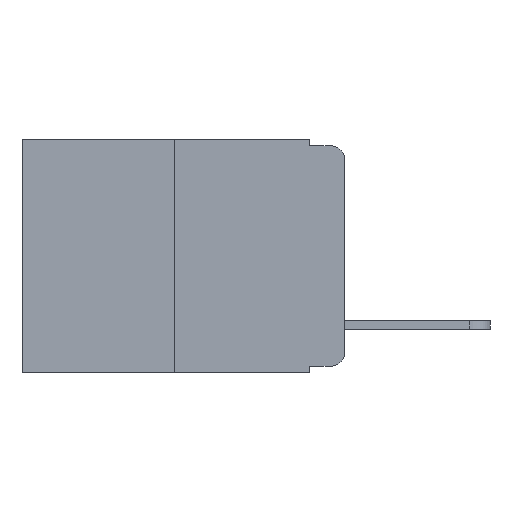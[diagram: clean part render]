
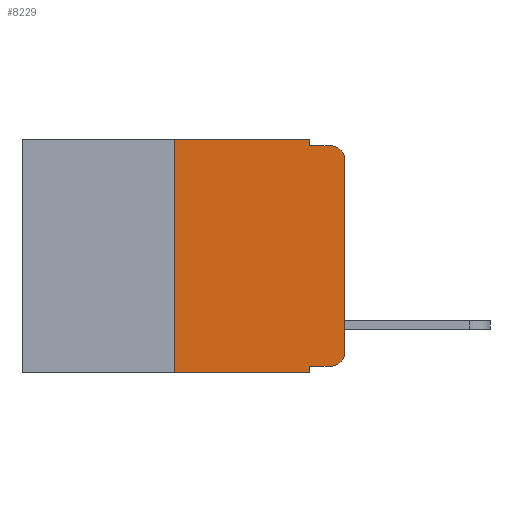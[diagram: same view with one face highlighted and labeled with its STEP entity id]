
A CAD part, left-side view. The second image highlights one B-rep face of the part: STEP entity #8229.
In plain terms, the highlighted planar face has unit normal (-1, 0, 0).
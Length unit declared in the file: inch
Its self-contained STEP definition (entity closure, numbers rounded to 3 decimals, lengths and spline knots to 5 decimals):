
#156 = EDGE_CURVE ( 'NONE', #7094, #14246, #8089, .T. ) ;
#465 = AXIS2_PLACEMENT_3D ( 'NONE', #5939, #7068, #10339 ) ;
#545 = VERTEX_POINT ( 'NONE', #8440 ) ;
#773 = CARTESIAN_POINT ( 'NONE',  ( 0., 0., -0.313 ) ) ;
#799 = VECTOR ( 'NONE', #7182, 39.37008 ) ;
#1074 = ORIENTED_EDGE ( 'NONE', *, *, #1769, .T. ) ;
#1079 = CARTESIAN_POINT ( 'NONE',  ( 0., 0.25, -0.343 ) ) ;
#1529 = EDGE_CURVE ( 'NONE', #7950, #545, #6477, .T. ) ;
#1769 = EDGE_CURVE ( 'NONE', #13994, #12586, #9266, .T. ) ;
#2109 = CARTESIAN_POINT ( 'NONE',  ( 0., 0.473, 0. ) ) ;
#2156 = DIRECTION ( 'NONE',  ( 0., -1., 0. ) ) ;
#2296 = LINE ( 'NONE', #3950, #11713 ) ;
#2600 = DIRECTION ( 'NONE',  ( 0., -1., 0. ) ) ;
#2976 = LINE ( 'NONE', #9887, #11186 ) ;
#3280 = DIRECTION ( 'NONE',  ( 0., 0., -1. ) ) ;
#3608 = DIRECTION ( 'NONE',  ( 0., 0., -1. ) ) ;
#3950 = CARTESIAN_POINT ( 'NONE',  ( 0., 0.25, 0. ) ) ;
#4275 = ORIENTED_EDGE ( 'NONE', *, *, #14229, .F. ) ;
#4282 = ORIENTED_EDGE ( 'NONE', *, *, #156, .F. ) ;
#4387 = CARTESIAN_POINT ( 'NONE',  ( 0., 0.051, 0. ) ) ;
#4635 = VERTEX_POINT ( 'NONE', #8736 ) ;
#4652 = EDGE_CURVE ( 'NONE', #545, #7094, #5763, .T. ) ;
#4872 = DIRECTION ( 'NONE',  ( 0., 0., 1. ) ) ;
#4906 = DIRECTION ( 'NONE',  ( 0., 0., 1. ) ) ;
#5021 = CARTESIAN_POINT ( 'NONE',  ( 0., 0.051, -0.333 ) ) ;
#5056 = EDGE_CURVE ( 'NONE', #12586, #4635, #2976, .T. ) ;
#5356 = PLANE ( 'NONE',  #9702 ) ;
#5615 = DIRECTION ( 'NONE',  ( 0., 0., -1. ) ) ;
#5763 = LINE ( 'NONE', #4387, #7341 ) ;
#5784 = CARTESIAN_POINT ( 'NONE',  ( 0., 0.02, -0.03 ) ) ;
#5939 = CARTESIAN_POINT ( 'NONE',  ( 0., 0.02, -0.313 ) ) ;
#6159 = ORIENTED_EDGE ( 'NONE', *, *, #5056, .T. ) ;
#6477 = LINE ( 'NONE', #2109, #11557 ) ;
#6562 = CARTESIAN_POINT ( 'NONE',  ( 0., 0.051, -0.343 ) ) ;
#6568 = ORIENTED_EDGE ( 'NONE', *, *, #7954, .T. ) ;
#6570 = EDGE_CURVE ( 'NONE', #4635, #14246, #12740, .T. ) ;
#7065 = VERTEX_POINT ( 'NONE', #6562 ) ;
#7068 = DIRECTION ( 'NONE',  ( -1., 0., 0. ) ) ;
#7094 = VERTEX_POINT ( 'NONE', #13340 ) ;
#7182 = DIRECTION ( 'NONE',  ( 0., -1., 0. ) ) ;
#7341 = VECTOR ( 'NONE', #11244, 39.37008 ) ;
#7663 = ORIENTED_EDGE ( 'NONE', *, *, #6570, .T. ) ;
#7739 = VECTOR ( 'NONE', #9499, 39.37008 ) ;
#7950 = VERTEX_POINT ( 'NONE', #9463 ) ;
#7954 = EDGE_CURVE ( 'NONE', #13174, #13994, #11627, .T. ) ;
#7962 = CARTESIAN_POINT ( 'NONE',  ( 0., 0.051, 0. ) ) ;
#8089 = LINE ( 'NONE', #10083, #10552 ) ;
#8229 = ADVANCED_FACE ( 'NONE', ( #10780 ), #5356, .F. ) ;
#8440 = CARTESIAN_POINT ( 'NONE',  ( 0., 0.051, 0. ) ) ;
#8736 = CARTESIAN_POINT ( 'NONE',  ( 0., 0., -0.03 ) ) ;
#8878 = ORIENTED_EDGE ( 'NONE', *, *, #1529, .F. ) ;
#9266 = CIRCLE ( 'NONE', #465, 0.02 ) ;
#9463 = CARTESIAN_POINT ( 'NONE',  ( 0., 0.25, 0. ) ) ;
#9477 = CARTESIAN_POINT ( 'NONE',  ( 0., 0.051, -0.333 ) ) ;
#9484 = AXIS2_PLACEMENT_3D ( 'NONE', #5784, #10283, #3608 ) ;
#9499 = DIRECTION ( 'NONE',  ( 0., -1., 0. ) ) ;
#9659 = VERTEX_POINT ( 'NONE', #1079 ) ;
#9702 = AXIS2_PLACEMENT_3D ( 'NONE', #9855, #14422, #3280 ) ;
#9855 = CARTESIAN_POINT ( 'NONE',  ( 0., 0.473, 0. ) ) ;
#9887 = CARTESIAN_POINT ( 'NONE',  ( 0., 0., 0. ) ) ;
#10083 = CARTESIAN_POINT ( 'NONE',  ( 0., 0.051, -0.01 ) ) ;
#10283 = DIRECTION ( 'NONE',  ( -1., 0., 0. ) ) ;
#10339 = DIRECTION ( 'NONE',  ( 0., 0., -1. ) ) ;
#10552 = VECTOR ( 'NONE', #2600, 39.37008 ) ;
#10780 = FACE_OUTER_BOUND ( 'NONE', #12236, .T. ) ;
#11186 = VECTOR ( 'NONE', #4872, 39.37008 ) ;
#11244 = DIRECTION ( 'NONE',  ( 0., 0., -1. ) ) ;
#11429 = EDGE_CURVE ( 'NONE', #13174, #7065, #12697, .T. ) ;
#11557 = VECTOR ( 'NONE', #2156, 39.37008 ) ;
#11627 = LINE ( 'NONE', #5021, #799 ) ;
#11713 = VECTOR ( 'NONE', #4906, 39.37008 ) ;
#12236 = EDGE_LOOP ( 'NONE', ( #6159, #7663, #4282, #14127, #8878, #4275, #13179, #14377, #6568, #1074 ) ) ;
#12431 = EDGE_CURVE ( 'NONE', #9659, #7065, #12493, .T. ) ;
#12493 = LINE ( 'NONE', #12562, #7739 ) ;
#12562 = CARTESIAN_POINT ( 'NONE',  ( 0., 0.473, -0.343 ) ) ;
#12565 = CARTESIAN_POINT ( 'NONE',  ( 0., 0.02, -0.333 ) ) ;
#12586 = VERTEX_POINT ( 'NONE', #773 ) ;
#12697 = LINE ( 'NONE', #7962, #13918 ) ;
#12740 = CIRCLE ( 'NONE', #9484, 0.02 ) ;
#13174 = VERTEX_POINT ( 'NONE', #9477 ) ;
#13179 = ORIENTED_EDGE ( 'NONE', *, *, #12431, .T. ) ;
#13340 = CARTESIAN_POINT ( 'NONE',  ( 0., 0.051, -0.01 ) ) ;
#13918 = VECTOR ( 'NONE', #5615, 39.37008 ) ;
#13994 = VERTEX_POINT ( 'NONE', #12565 ) ;
#14127 = ORIENTED_EDGE ( 'NONE', *, *, #4652, .F. ) ;
#14167 = CARTESIAN_POINT ( 'NONE',  ( 0., 0.02, -0.01 ) ) ;
#14229 = EDGE_CURVE ( 'NONE', #9659, #7950, #2296, .T. ) ;
#14246 = VERTEX_POINT ( 'NONE', #14167 ) ;
#14377 = ORIENTED_EDGE ( 'NONE', *, *, #11429, .F. ) ;
#14422 = DIRECTION ( 'NONE',  ( 1., 0., 0. ) ) ;
